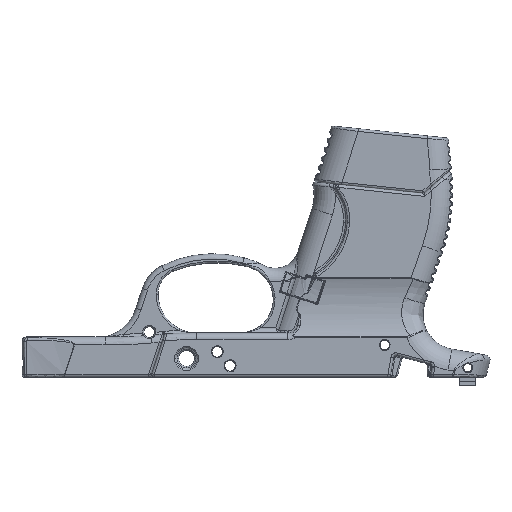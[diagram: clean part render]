
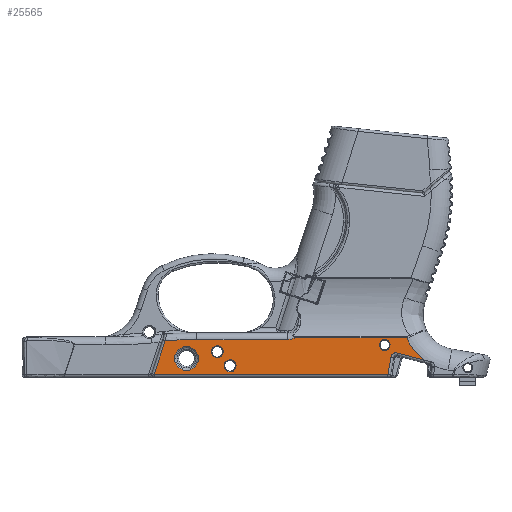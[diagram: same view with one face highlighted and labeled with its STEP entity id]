
A CAD part, front view. The second image highlights one B-rep face of the part: STEP entity #25565.
In plain terms, the highlighted planar face has unit normal (0, -1, 0).
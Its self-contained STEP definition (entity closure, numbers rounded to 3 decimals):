
#36=FACE_BOUND('',#4132,.T.);
#37=FACE_BOUND('',#4133,.T.);
#38=FACE_BOUND('',#4134,.T.);
#39=FACE_BOUND('',#4135,.T.);
#1364=PLANE('',#28081);
#2417=FACE_OUTER_BOUND('',#4131,.T.);
#4131=EDGE_LOOP('',(#20651,#20652,#20653,#20654,#20655,#20656,#20657,#20658,
#20659,#20660));
#4132=EDGE_LOOP('',(#20661));
#4133=EDGE_LOOP('',(#20662));
#4134=EDGE_LOOP('',(#20663));
#4135=EDGE_LOOP('',(#20664));
#5757=CIRCLE('',#27976,2.);
#5819=CIRCLE('',#28079,21.);
#5820=CIRCLE('',#28082,6.5);
#5821=CIRCLE('',#28083,193.385);
#5822=CIRCLE('',#28084,2.);
#5823=CIRCLE('',#28085,2.25);
#5824=CIRCLE('',#28086,4.5);
#5825=CIRCLE('',#28087,2.25);
#7264=LINE('',#55472,#8512);
#7265=LINE('',#55483,#8513);
#7270=LINE('',#55617,#8518);
#7300=LINE('',#55989,#8548);
#7303=LINE('',#56019,#8551);
#7304=LINE('',#56023,#8552);
#8512=VECTOR('',#33354,10.);
#8513=VECTOR('',#33367,10.);
#8518=VECTOR('',#33408,10.);
#8548=VECTOR('',#33590,10.);
#8551=VECTOR('',#33609,10.);
#8552=VECTOR('',#33612,10.);
#11300=VERTEX_POINT('',#55465);
#11303=VERTEX_POINT('',#55470);
#11305=VERTEX_POINT('',#55475);
#11307=VERTEX_POINT('',#55481);
#11317=VERTEX_POINT('',#55614);
#11369=VERTEX_POINT('',#55988);
#11374=VERTEX_POINT('',#56007);
#11376=VERTEX_POINT('',#56018);
#11377=VERTEX_POINT('',#56020);
#11378=VERTEX_POINT('',#56022);
#11379=VERTEX_POINT('',#56025);
#11380=VERTEX_POINT('',#56027);
#11381=VERTEX_POINT('',#56029);
#11382=VERTEX_POINT('',#56031);
#14477=EDGE_CURVE('',#11303,#11300,#7264,.T.);
#14479=EDGE_CURVE('',#11305,#11303,#5757,.T.);
#14482=EDGE_CURVE('',#11307,#11305,#7265,.T.);
#14502=EDGE_CURVE('',#11300,#11317,#7270,.T.);
#14592=EDGE_CURVE('',#11317,#11369,#7300,.T.);
#14599=EDGE_CURVE('',#11374,#11307,#5819,.T.);
#14602=EDGE_CURVE('',#11376,#11374,#7303,.T.);
#14603=EDGE_CURVE('',#11377,#11376,#5820,.T.);
#14604=EDGE_CURVE('',#11378,#11377,#7304,.T.);
#14605=EDGE_CURVE('',#11369,#11378,#5821,.T.);
#14606=EDGE_CURVE('',#11379,#11379,#5822,.T.);
#14607=EDGE_CURVE('',#11380,#11380,#5823,.T.);
#14608=EDGE_CURVE('',#11381,#11381,#5824,.T.);
#14609=EDGE_CURVE('',#11382,#11382,#5825,.T.);
#20651=ORIENTED_EDGE('',*,*,#14502,.F.);
#20652=ORIENTED_EDGE('',*,*,#14477,.F.);
#20653=ORIENTED_EDGE('',*,*,#14479,.F.);
#20654=ORIENTED_EDGE('',*,*,#14482,.F.);
#20655=ORIENTED_EDGE('',*,*,#14599,.F.);
#20656=ORIENTED_EDGE('',*,*,#14602,.F.);
#20657=ORIENTED_EDGE('',*,*,#14603,.F.);
#20658=ORIENTED_EDGE('',*,*,#14604,.F.);
#20659=ORIENTED_EDGE('',*,*,#14605,.F.);
#20660=ORIENTED_EDGE('',*,*,#14592,.F.);
#20661=ORIENTED_EDGE('',*,*,#14606,.F.);
#20662=ORIENTED_EDGE('',*,*,#14607,.F.);
#20663=ORIENTED_EDGE('',*,*,#14608,.F.);
#20664=ORIENTED_EDGE('',*,*,#14609,.F.);
#25565=ADVANCED_FACE('',(#2417,#36,#37,#38,#39),#1364,.F.);
#27976=AXIS2_PLACEMENT_3D('',#55477,#33359,#33360);
#28079=AXIS2_PLACEMENT_3D('',#56012,#33601,#33602);
#28081=AXIS2_PLACEMENT_3D('',#56017,#33607,#33608);
#28082=AXIS2_PLACEMENT_3D('',#56021,#33610,#33611);
#28083=AXIS2_PLACEMENT_3D('',#56024,#33613,#33614);
#28084=AXIS2_PLACEMENT_3D('',#56026,#33615,#33616);
#28085=AXIS2_PLACEMENT_3D('',#56028,#33617,#33618);
#28086=AXIS2_PLACEMENT_3D('',#56030,#33619,#33620);
#28087=AXIS2_PLACEMENT_3D('',#56032,#33621,#33622);
#33354=DIRECTION('',(-0.174,0.,-0.985));
#33359=DIRECTION('center_axis',(0.,-1.,0.));
#33360=DIRECTION('ref_axis',(-0.537,0.,0.843));
#33367=DIRECTION('',(-0.966,0.,0.259));
#33408=DIRECTION('',(-1.,0.,0.));
#33590=DIRECTION('',(0.309,0.,0.951));
#33601=DIRECTION('center_axis',(0.,-1.,0.));
#33602=DIRECTION('ref_axis',(-0.492,0.,-0.871));
#33607=DIRECTION('center_axis',(0.,1.,0.));
#33608=DIRECTION('ref_axis',(1.,0.,0.));
#33609=DIRECTION('',(1.,0.,0.));
#33610=DIRECTION('center_axis',(0.,-1.,0.));
#33611=DIRECTION('ref_axis',(0.588,0.,-0.809));
#33612=DIRECTION('',(1.,0.,0.));
#33613=DIRECTION('center_axis',(0.,1.,0.));
#33614=DIRECTION('ref_axis',(-0.031,0.,1.));
#33615=DIRECTION('center_axis',(0.,-1.,0.));
#33616=DIRECTION('ref_axis',(1.,0.,0.));
#33617=DIRECTION('center_axis',(0.,-1.,0.));
#33618=DIRECTION('ref_axis',(1.,0.,0.));
#33619=DIRECTION('center_axis',(0.,-1.,0.));
#33620=DIRECTION('ref_axis',(1.,0.,0.));
#33621=DIRECTION('center_axis',(0.,-1.,0.));
#33622=DIRECTION('ref_axis',(1.,0.,0.));
#55465=CARTESIAN_POINT('',(60.55,-15.,-39.));
#55470=CARTESIAN_POINT('',(61.682,-15.,-32.58));
#55472=CARTESIAN_POINT('',(63.155,-15.,-24.223));
#55475=CARTESIAN_POINT('',(64.169,-15.,-30.996));
#55477=CARTESIAN_POINT('Origin',(63.651,-15.,-32.927));
#55481=CARTESIAN_POINT('',(74.299,-15.,-33.71));
#55483=CARTESIAN_POINT('',(35.838,-15.,-23.404));
#55614=CARTESIAN_POINT('',(-26.624,-15.,-39.));
#55617=CARTESIAN_POINT('',(52.3,-15.,-39.));
#55988=CARTESIAN_POINT('',(-22.516,-15.,-26.358));
#55989=CARTESIAN_POINT('',(-17.072,-15.,-9.602));
#56007=CARTESIAN_POINT('',(67.471,-15.,-25.272));
#56012=CARTESIAN_POINT('Origin',(86.655,-15.,-16.73));
#56017=CARTESIAN_POINT('Origin',(9.6,-15.,1.309));
#56018=CARTESIAN_POINT('',(26.047,-15.,-25.272));
#56019=CARTESIAN_POINT('',(110.,-15.,-25.272));
#56020=CARTESIAN_POINT('',(23.058,-15.,-26.));
#56021=CARTESIAN_POINT('Origin',(23.058,-15.,-19.5));
#56022=CARTESIAN_POINT('',(-10.75,-15.,-26.));
#56023=CARTESIAN_POINT('',(7.425,-15.,-26.));
#56024=CARTESIAN_POINT('Origin',(-10.75,-15.,-219.385));
#56025=CARTESIAN_POINT('',(57.375,-15.,-28.));
#56026=CARTESIAN_POINT('Origin',(59.375,-15.,-28.));
#56027=CARTESIAN_POINT('',(-5.35,-15.,-30.525));
#56028=CARTESIAN_POINT('Origin',(-3.1,-15.,-30.525));
#56029=CARTESIAN_POINT('',(-19.1,-15.,-33.025));
#56030=CARTESIAN_POINT('Origin',(-14.6,-15.,-33.025));
#56031=CARTESIAN_POINT('',(-0.6,-15.,-35.775));
#56032=CARTESIAN_POINT('Origin',(1.65,-15.,-35.775));
